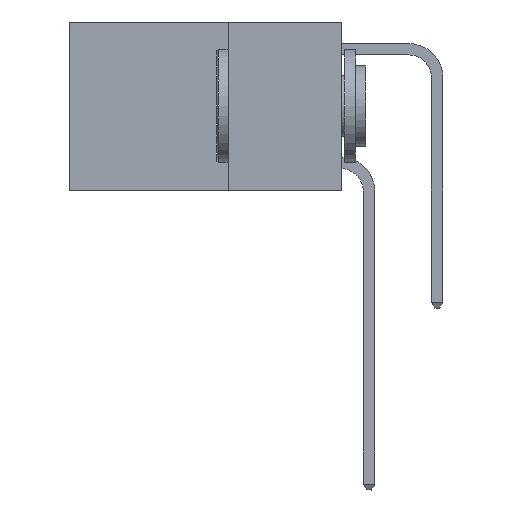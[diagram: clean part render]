
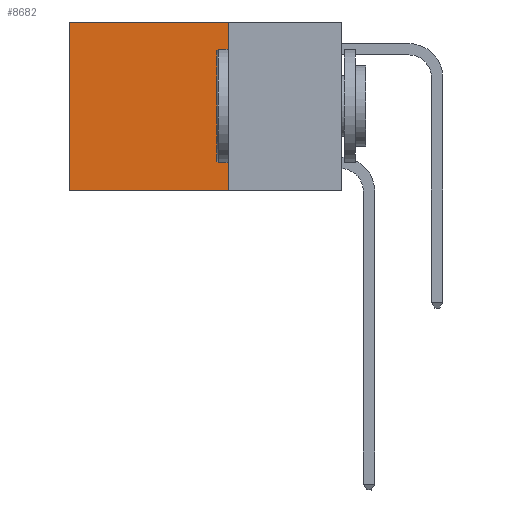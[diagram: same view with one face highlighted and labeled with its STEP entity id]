
A CAD part, left-side view. The second image highlights one B-rep face of the part: STEP entity #8682.
In plain terms, the highlighted planar face has unit normal (-1, 0, 0).
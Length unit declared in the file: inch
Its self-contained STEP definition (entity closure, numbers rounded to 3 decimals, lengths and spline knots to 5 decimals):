
#1209 = EDGE_CURVE ( 'NONE', #14156, #24463, #24069, .T. ) ;
#1506 = ORIENTED_EDGE ( 'NONE', *, *, #15909, .T. ) ;
#1914 = DIRECTION ( 'NONE',  ( 0., 0., -1. ) ) ;
#3806 = VERTEX_POINT ( 'NONE', #12995 ) ;
#4141 = CARTESIAN_POINT ( 'NONE',  ( 0.2625, 0.25, 0. ) ) ;
#4982 = ORIENTED_EDGE ( 'NONE', *, *, #28807, .F. ) ;
#5585 = CARTESIAN_POINT ( 'NONE',  ( 0.2625, 0.25, -0.37 ) ) ;
#5766 = VECTOR ( 'NONE', #19636, 39.37008 ) ;
#6355 = PLANE ( 'NONE',  #23791 ) ;
#6644 = CARTESIAN_POINT ( 'NONE',  ( 0.2625, 0.25, -0.37 ) ) ;
#6984 = LINE ( 'NONE', #22527, #8240 ) ;
#7822 = EDGE_LOOP ( 'NONE', ( #1506, #23227, #4982, #12880 ) ) ;
#8240 = VECTOR ( 'NONE', #26813, 39.37008 ) ;
#8544 = LINE ( 'NONE', #17575, #11149 ) ;
#8682 = ADVANCED_FACE ( 'NONE', ( #24417 ), #6355, .F. ) ;
#9324 = VERTEX_POINT ( 'NONE', #14560 ) ;
#10499 = DIRECTION ( 'NONE',  ( 1., 0., 0. ) ) ;
#10598 = EDGE_CURVE ( 'NONE', #3806, #9324, #28068, .T. ) ;
#11149 = VECTOR ( 'NONE', #26589, 39.37008 ) ;
#12880 = ORIENTED_EDGE ( 'NONE', *, *, #10598, .T. ) ;
#12995 = CARTESIAN_POINT ( 'NONE',  ( 0.2625, 0.25, 0. ) ) ;
#14156 = VERTEX_POINT ( 'NONE', #6644 ) ;
#14560 = CARTESIAN_POINT ( 'NONE',  ( 0.2625, 0.6, 0. ) ) ;
#15812 = CARTESIAN_POINT ( 'NONE',  ( 0.2625, 0.6, -0.37 ) ) ;
#15909 = EDGE_CURVE ( 'NONE', #9324, #24463, #8544, .T. ) ;
#17575 = CARTESIAN_POINT ( 'NONE',  ( 0.2625, 0.6, 0. ) ) ;
#19636 = DIRECTION ( 'NONE',  ( 0., 1., 0. ) ) ;
#20533 = VECTOR ( 'NONE', #20700, 39.37008 ) ;
#20700 = DIRECTION ( 'NONE',  ( 0., 1., 0. ) ) ;
#22527 = CARTESIAN_POINT ( 'NONE',  ( 0.2625, 0.25, 0. ) ) ;
#23227 = ORIENTED_EDGE ( 'NONE', *, *, #1209, .F. ) ;
#23625 = CARTESIAN_POINT ( 'NONE',  ( 0.2625, 0.25, 0. ) ) ;
#23791 = AXIS2_PLACEMENT_3D ( 'NONE', #4141, #10499, #1914 ) ;
#24069 = LINE ( 'NONE', #5585, #5766 ) ;
#24417 = FACE_OUTER_BOUND ( 'NONE', #7822, .T. ) ;
#24463 = VERTEX_POINT ( 'NONE', #15812 ) ;
#26589 = DIRECTION ( 'NONE',  ( 0., 0., -1. ) ) ;
#26813 = DIRECTION ( 'NONE',  ( 0., 0., -1. ) ) ;
#28068 = LINE ( 'NONE', #23625, #20533 ) ;
#28807 = EDGE_CURVE ( 'NONE', #3806, #14156, #6984, .T. ) ;
